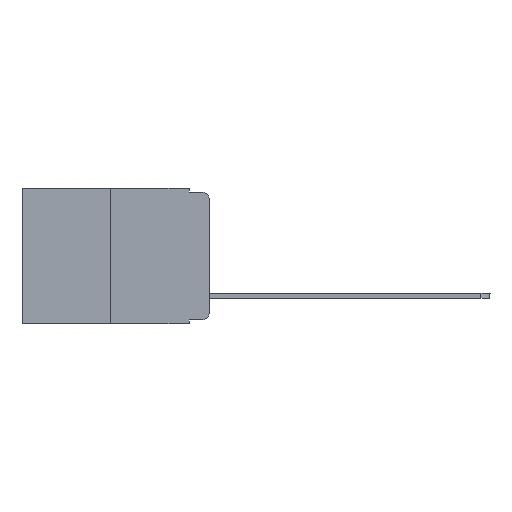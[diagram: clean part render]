
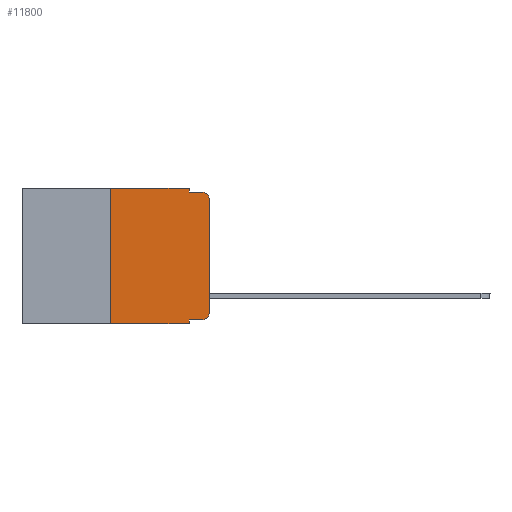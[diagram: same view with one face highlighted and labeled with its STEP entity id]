
A CAD part, left-side view. The second image highlights one B-rep face of the part: STEP entity #11800.
In plain terms, the highlighted planar face has unit normal (-1, 0, 0).
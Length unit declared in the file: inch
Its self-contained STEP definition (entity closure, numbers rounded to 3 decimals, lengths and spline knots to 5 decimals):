
#276 = VERTEX_POINT ( 'NONE', #11068 ) ;
#283 = CARTESIAN_POINT ( 'NONE',  ( 0., 0.051, -0.333 ) ) ;
#401 = VERTEX_POINT ( 'NONE', #4364 ) ;
#425 = CARTESIAN_POINT ( 'NONE',  ( 0., 0.051, 0. ) ) ;
#498 = CARTESIAN_POINT ( 'NONE',  ( 0., 0., -0.03 ) ) ;
#613 = DIRECTION ( 'NONE',  ( -1., 0., 0. ) ) ;
#710 = CARTESIAN_POINT ( 'NONE',  ( 0., 0., -0.313 ) ) ;
#750 = EDGE_CURVE ( 'NONE', #4203, #2876, #7352, .T. ) ;
#791 = CARTESIAN_POINT ( 'NONE',  ( 0., 0.02, -0.01 ) ) ;
#794 = CARTESIAN_POINT ( 'NONE',  ( 0., 0., 0. ) ) ;
#889 = EDGE_CURVE ( 'NONE', #401, #8497, #12011, .T. ) ;
#911 = DIRECTION ( 'NONE',  ( -1., 0., 0. ) ) ;
#954 = ORIENTED_EDGE ( 'NONE', *, *, #9987, .F. ) ;
#1001 = ORIENTED_EDGE ( 'NONE', *, *, #889, .F. ) ;
#1111 = ORIENTED_EDGE ( 'NONE', *, *, #4081, .T. ) ;
#1334 = CARTESIAN_POINT ( 'NONE',  ( 0., 0.051, 0. ) ) ;
#1387 = LINE ( 'NONE', #283, #4867 ) ;
#1653 = EDGE_CURVE ( 'NONE', #3194, #6028, #5529, .T. ) ;
#1935 = CARTESIAN_POINT ( 'NONE',  ( 0., 0.02, -0.03 ) ) ;
#2034 = VECTOR ( 'NONE', #3686, 39.37008 ) ;
#2076 = VECTOR ( 'NONE', #8521, 39.37008 ) ;
#2137 = CARTESIAN_POINT ( 'NONE',  ( 0., 0.051, -0.343 ) ) ;
#2373 = ORIENTED_EDGE ( 'NONE', *, *, #5172, .F. ) ;
#2518 = ORIENTED_EDGE ( 'NONE', *, *, #11622, .F. ) ;
#2684 = DIRECTION ( 'NONE',  ( 1., 0., 0. ) ) ;
#2876 = VERTEX_POINT ( 'NONE', #2137 ) ;
#3193 = DIRECTION ( 'NONE',  ( 0., -1., 0. ) ) ;
#3194 = VERTEX_POINT ( 'NONE', #710 ) ;
#3452 = AXIS2_PLACEMENT_3D ( 'NONE', #1935, #911, #11831 ) ;
#3593 = CARTESIAN_POINT ( 'NONE',  ( 0., 0.473, 0. ) ) ;
#3686 = DIRECTION ( 'NONE',  ( 0., 0., -1. ) ) ;
#3731 = EDGE_CURVE ( 'NONE', #276, #2876, #5812, .T. ) ;
#3909 = VECTOR ( 'NONE', #10368, 39.37008 ) ;
#4081 = EDGE_CURVE ( 'NONE', #4203, #11976, #1387, .T. ) ;
#4198 = DIRECTION ( 'NONE',  ( 0., -1., 0. ) ) ;
#4200 = EDGE_CURVE ( 'NONE', #11976, #3194, #12314, .T. ) ;
#4203 = VERTEX_POINT ( 'NONE', #8633 ) ;
#4305 = AXIS2_PLACEMENT_3D ( 'NONE', #3593, #2684, #5579 ) ;
#4364 = CARTESIAN_POINT ( 'NONE',  ( 0., 0.25, 0. ) ) ;
#4398 = CARTESIAN_POINT ( 'NONE',  ( 0., 0.473, 0. ) ) ;
#4691 = DIRECTION ( 'NONE',  ( 0., 0., 1. ) ) ;
#4867 = VECTOR ( 'NONE', #4198, 39.37008 ) ;
#5172 = EDGE_CURVE ( 'NONE', #8497, #5371, #7870, .T. ) ;
#5180 = CARTESIAN_POINT ( 'NONE',  ( 0., 0.473, -0.343 ) ) ;
#5371 = VERTEX_POINT ( 'NONE', #5970 ) ;
#5529 = LINE ( 'NONE', #794, #8953 ) ;
#5579 = DIRECTION ( 'NONE',  ( 0., 0., -1. ) ) ;
#5812 = LINE ( 'NONE', #5180, #6898 ) ;
#5879 = CARTESIAN_POINT ( 'NONE',  ( 0., 0.051, 0. ) ) ;
#5970 = CARTESIAN_POINT ( 'NONE',  ( 0., 0.051, -0.01 ) ) ;
#6028 = VERTEX_POINT ( 'NONE', #498 ) ;
#6152 = ORIENTED_EDGE ( 'NONE', *, *, #1653, .T. ) ;
#6258 = VECTOR ( 'NONE', #7334, 39.37008 ) ;
#6640 = CARTESIAN_POINT ( 'NONE',  ( 0., 0.02, -0.313 ) ) ;
#6898 = VECTOR ( 'NONE', #3193, 39.37008 ) ;
#6900 = ORIENTED_EDGE ( 'NONE', *, *, #3731, .T. ) ;
#7334 = DIRECTION ( 'NONE',  ( 0., -1., 0. ) ) ;
#7352 = LINE ( 'NONE', #5879, #2034 ) ;
#7443 = EDGE_CURVE ( 'NONE', #6028, #11208, #7572, .T. ) ;
#7572 = CIRCLE ( 'NONE', #3452, 0.02 ) ;
#7627 = DIRECTION ( 'NONE',  ( 0., 0., -1. ) ) ;
#7796 = ORIENTED_EDGE ( 'NONE', *, *, #4200, .T. ) ;
#7870 = LINE ( 'NONE', #1334, #9735 ) ;
#8254 = LINE ( 'NONE', #12395, #3909 ) ;
#8497 = VERTEX_POINT ( 'NONE', #425 ) ;
#8504 = CARTESIAN_POINT ( 'NONE',  ( 0., 0.02, -0.333 ) ) ;
#8521 = DIRECTION ( 'NONE',  ( 0., 0., 1. ) ) ;
#8633 = CARTESIAN_POINT ( 'NONE',  ( 0., 0.051, -0.333 ) ) ;
#8728 = FACE_OUTER_BOUND ( 'NONE', #9165, .T. ) ;
#8953 = VECTOR ( 'NONE', #4691, 39.37008 ) ;
#9165 = EDGE_LOOP ( 'NONE', ( #6152, #12639, #2518, #2373, #1001, #954, #6900, #12660, #1111, #7796 ) ) ;
#9405 = LINE ( 'NONE', #9463, #2076 ) ;
#9463 = CARTESIAN_POINT ( 'NONE',  ( 0., 0.25, 0. ) ) ;
#9735 = VECTOR ( 'NONE', #11444, 39.37008 ) ;
#9987 = EDGE_CURVE ( 'NONE', #276, #401, #9405, .T. ) ;
#10368 = DIRECTION ( 'NONE',  ( 0., -1., 0. ) ) ;
#11068 = CARTESIAN_POINT ( 'NONE',  ( 0., 0.25, -0.343 ) ) ;
#11208 = VERTEX_POINT ( 'NONE', #791 ) ;
#11444 = DIRECTION ( 'NONE',  ( 0., 0., -1. ) ) ;
#11622 = EDGE_CURVE ( 'NONE', #5371, #11208, #8254, .T. ) ;
#11776 = AXIS2_PLACEMENT_3D ( 'NONE', #6640, #613, #7627 ) ;
#11800 = ADVANCED_FACE ( 'NONE', ( #8728 ), #12575, .F. ) ;
#11831 = DIRECTION ( 'NONE',  ( 0., 0., -1. ) ) ;
#11976 = VERTEX_POINT ( 'NONE', #8504 ) ;
#12011 = LINE ( 'NONE', #4398, #6258 ) ;
#12314 = CIRCLE ( 'NONE', #11776, 0.02 ) ;
#12395 = CARTESIAN_POINT ( 'NONE',  ( 0., 0.051, -0.01 ) ) ;
#12575 = PLANE ( 'NONE',  #4305 ) ;
#12639 = ORIENTED_EDGE ( 'NONE', *, *, #7443, .T. ) ;
#12660 = ORIENTED_EDGE ( 'NONE', *, *, #750, .F. ) ;
